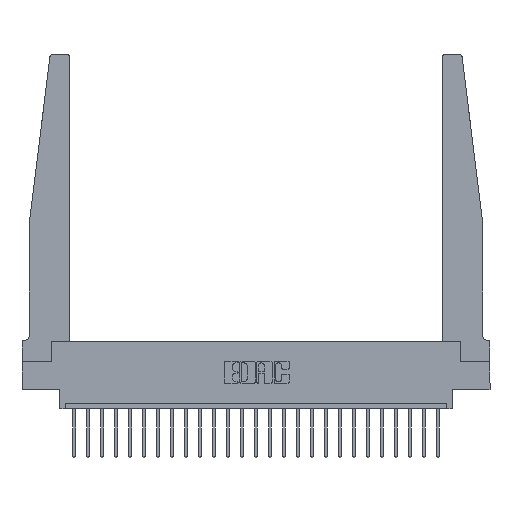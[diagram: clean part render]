
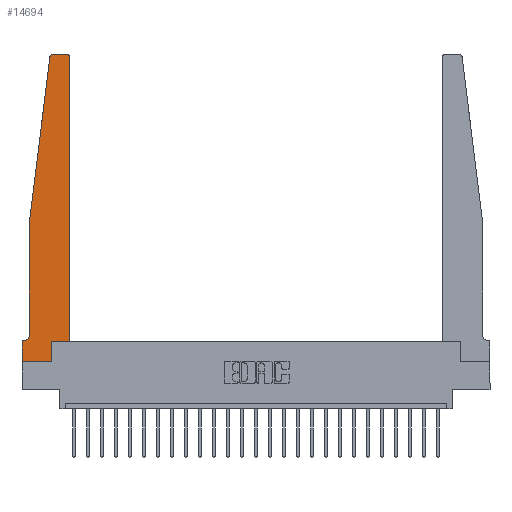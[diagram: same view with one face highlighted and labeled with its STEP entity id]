
A CAD part, top view. The second image highlights one B-rep face of the part: STEP entity #14694.
In plain terms, the highlighted planar face has unit normal (0, 0, 1).
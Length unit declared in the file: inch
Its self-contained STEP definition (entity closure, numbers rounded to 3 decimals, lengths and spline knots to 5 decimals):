
#19 = VECTOR ( 'NONE', #10555, 39.37008 ) ;
#277 = CIRCLE ( 'NONE', #19754, 0.03 ) ;
#349 = DIRECTION ( 'NONE',  ( 1., 0., 0. ) ) ;
#543 = VECTOR ( 'NONE', #22167, 39.37008 ) ;
#785 = VERTEX_POINT ( 'NONE', #1982 ) ;
#990 = EDGE_CURVE ( 'NONE', #1516, #7940, #18161, .T. ) ;
#1516 = VERTEX_POINT ( 'NONE', #2194 ) ;
#1815 = VECTOR ( 'NONE', #2625, 39.37008 ) ;
#1857 = ORIENTED_EDGE ( 'NONE', *, *, #6208, .T. ) ;
#1933 = EDGE_CURVE ( 'NONE', #7724, #15888, #16276, .T. ) ;
#1951 = VECTOR ( 'NONE', #15470, 39.37008 ) ;
#1982 = CARTESIAN_POINT ( 'NONE',  ( 0.2605, 0., 0.37 ) ) ;
#2194 = CARTESIAN_POINT ( 'NONE',  ( 0.24675, 2.72367, 0.37 ) ) ;
#2307 = CARTESIAN_POINT ( 'NONE',  ( 0.065, 0.2375, 0.37 ) ) ;
#2308 = VERTEX_POINT ( 'NONE', #15881 ) ;
#2516 = EDGE_CURVE ( 'NONE', #14192, #1516, #277, .T. ) ;
#2606 = VERTEX_POINT ( 'NONE', #7163 ) ;
#2625 = DIRECTION ( 'NONE',  ( 1., 0., 0. ) ) ;
#3094 = VECTOR ( 'NONE', #7414, 39.37008 ) ;
#3252 = VERTEX_POINT ( 'NONE', #14813 ) ;
#3299 = LINE ( 'NONE', #4802, #7540 ) ;
#4029 = CARTESIAN_POINT ( 'NONE',  ( 0.395, 2.72, 0.37 ) ) ;
#4125 = FACE_OUTER_BOUND ( 'NONE', #15138, .T. ) ;
#4237 = DIRECTION ( 'NONE',  ( 0., 0., 1. ) ) ;
#4622 = ORIENTED_EDGE ( 'NONE', *, *, #7421, .T. ) ;
#4802 = CARTESIAN_POINT ( 'NONE',  ( 0., 0., 0.37 ) ) ;
#5341 = CARTESIAN_POINT ( 'NONE',  ( 0.2605, 0.18, 0.37 ) ) ;
#5442 = CARTESIAN_POINT ( 'NONE',  ( 0.065, 1.25, 0.37 ) ) ;
#5846 = EDGE_CURVE ( 'NONE', #19757, #7386, #12205, .T. ) ;
#6142 = DIRECTION ( 'NONE',  ( 0., 0., 1. ) ) ;
#6175 = CARTESIAN_POINT ( 'NONE',  ( 0.425, 0.18, 0.37 ) ) ;
#6208 = EDGE_CURVE ( 'NONE', #785, #2308, #22017, .T. ) ;
#6301 = EDGE_CURVE ( 'NONE', #3252, #785, #3299, .T. ) ;
#6676 = CARTESIAN_POINT ( 'NONE',  ( 0.015, 0.2375, 0.37 ) ) ;
#6791 = CARTESIAN_POINT ( 'NONE',  ( 0.015, 0.1875, 0.37 ) ) ;
#7163 = CARTESIAN_POINT ( 'NONE',  ( 0.425, 0.18, 0.37 ) ) ;
#7386 = VERTEX_POINT ( 'NONE', #22641 ) ;
#7414 = DIRECTION ( 'NONE',  ( 0., -1., 0. ) ) ;
#7421 = EDGE_CURVE ( 'NONE', #7386, #14192, #17842, .T. ) ;
#7540 = VECTOR ( 'NONE', #10773, 39.37008 ) ;
#7724 = VERTEX_POINT ( 'NONE', #2307 ) ;
#7890 = LINE ( 'NONE', #6175, #1951 ) ;
#7940 = VERTEX_POINT ( 'NONE', #14740 ) ;
#7953 = CARTESIAN_POINT ( 'NONE',  ( 0., 0., 0.37 ) ) ;
#8320 = AXIS2_PLACEMENT_3D ( 'NONE', #4029, #6142, #349 ) ;
#8621 = LINE ( 'NONE', #23594, #19 ) ;
#9028 = EDGE_CURVE ( 'NONE', #2606, #19757, #7890, .T. ) ;
#9284 = ORIENTED_EDGE ( 'NONE', *, *, #15516, .T. ) ;
#10065 = CARTESIAN_POINT ( 'NONE',  ( 0.25, 2.75, 0.37 ) ) ;
#10069 = CARTESIAN_POINT ( 'NONE',  ( 0., 0.1875, 0.37 ) ) ;
#10121 = DIRECTION ( 'NONE',  ( 1., 0., 0. ) ) ;
#10127 = ORIENTED_EDGE ( 'NONE', *, *, #990, .T. ) ;
#10555 = DIRECTION ( 'NONE',  ( -1., 0., 0. ) ) ;
#10666 = CARTESIAN_POINT ( 'NONE',  ( 0.27653, 2.75, 0.37 ) ) ;
#10773 = DIRECTION ( 'NONE',  ( 1., 0., 0. ) ) ;
#11436 = LINE ( 'NONE', #5442, #3094 ) ;
#11594 = LINE ( 'NONE', #7953, #543 ) ;
#11933 = EDGE_CURVE ( 'NONE', #19007, #3252, #11594, .T. ) ;
#11956 = LINE ( 'NONE', #19338, #1815 ) ;
#12205 = CIRCLE ( 'NONE', #8320, 0.03 ) ;
#12434 = DIRECTION ( 'NONE',  ( 0., 0., 1. ) ) ;
#12809 = CARTESIAN_POINT ( 'NONE',  ( 0.425, 2.72, 0.37 ) ) ;
#14042 = CARTESIAN_POINT ( 'NONE',  ( 0., 0.1875, 0.37 ) ) ;
#14192 = VERTEX_POINT ( 'NONE', #10666 ) ;
#14674 = ORIENTED_EDGE ( 'NONE', *, *, #5846, .T. ) ;
#14694 = ADVANCED_FACE ( 'NONE', ( #4125 ), #17672, .T. ) ;
#14740 = CARTESIAN_POINT ( 'NONE',  ( 0.065, 1.25, 0.37 ) ) ;
#14813 = CARTESIAN_POINT ( 'NONE',  ( 0., 0., 0.37 ) ) ;
#15138 = EDGE_LOOP ( 'NONE', ( #4622, #15188, #10127, #16467, #22229, #19862, #21966, #17413, #1857, #9284, #16866, #14674 ) ) ;
#15188 = ORIENTED_EDGE ( 'NONE', *, *, #2516, .T. ) ;
#15470 = DIRECTION ( 'NONE',  ( 0., 1., 0. ) ) ;
#15516 = EDGE_CURVE ( 'NONE', #2308, #2606, #11956, .T. ) ;
#15881 = CARTESIAN_POINT ( 'NONE',  ( 0.2605, 0.18, 0.37 ) ) ;
#15888 = VERTEX_POINT ( 'NONE', #6791 ) ;
#15936 = DIRECTION ( 'NONE',  ( -1., 0., 0. ) ) ;
#16076 = DIRECTION ( 'NONE',  ( -1., 0., 0. ) ) ;
#16276 = CIRCLE ( 'NONE', #20494, 0.05 ) ;
#16467 = ORIENTED_EDGE ( 'NONE', *, *, #16974, .T. ) ;
#16488 = CARTESIAN_POINT ( 'NONE',  ( 0.065, 1.25, 0.37 ) ) ;
#16866 = ORIENTED_EDGE ( 'NONE', *, *, #9028, .T. ) ;
#16974 = EDGE_CURVE ( 'NONE', #7940, #7724, #11436, .T. ) ;
#17413 = ORIENTED_EDGE ( 'NONE', *, *, #6301, .T. ) ;
#17425 = AXIS2_PLACEMENT_3D ( 'NONE', #14042, #4237, #10121 ) ;
#17672 = PLANE ( 'NONE',  #17425 ) ;
#17842 = LINE ( 'NONE', #10065, #20212 ) ;
#18127 = DIRECTION ( 'NONE',  ( 1., 0., 0. ) ) ;
#18161 = LINE ( 'NONE', #16488, #20071 ) ;
#18291 = EDGE_CURVE ( 'NONE', #15888, #19007, #8621, .T. ) ;
#18406 = DIRECTION ( 'NONE',  ( -0.122, -0.992, 0. ) ) ;
#19007 = VERTEX_POINT ( 'NONE', #10069 ) ;
#19338 = CARTESIAN_POINT ( 'NONE',  ( 0.425, 0.18, 0.37 ) ) ;
#19754 = AXIS2_PLACEMENT_3D ( 'NONE', #24000, #12434, #18127 ) ;
#19757 = VERTEX_POINT ( 'NONE', #12809 ) ;
#19862 = ORIENTED_EDGE ( 'NONE', *, *, #18291, .T. ) ;
#20022 = DIRECTION ( 'NONE',  ( 0., 0., -1. ) ) ;
#20071 = VECTOR ( 'NONE', #18406, 39.37008 ) ;
#20212 = VECTOR ( 'NONE', #15936, 39.37008 ) ;
#20494 = AXIS2_PLACEMENT_3D ( 'NONE', #6676, #20022, #16076 ) ;
#21966 = ORIENTED_EDGE ( 'NONE', *, *, #11933, .T. ) ;
#22017 = LINE ( 'NONE', #5341, #23489 ) ;
#22167 = DIRECTION ( 'NONE',  ( 0., -1., 0. ) ) ;
#22229 = ORIENTED_EDGE ( 'NONE', *, *, #1933, .T. ) ;
#22478 = DIRECTION ( 'NONE',  ( 0., 1., 0. ) ) ;
#22641 = CARTESIAN_POINT ( 'NONE',  ( 0.395, 2.75, 0.37 ) ) ;
#23489 = VECTOR ( 'NONE', #22478, 39.37008 ) ;
#23594 = CARTESIAN_POINT ( 'NONE',  ( 0.065, 0.1875, 0.37 ) ) ;
#24000 = CARTESIAN_POINT ( 'NONE',  ( 0.27653, 2.72, 0.37 ) ) ;
